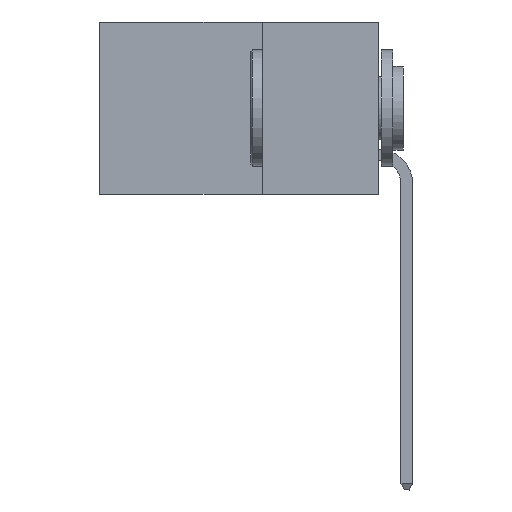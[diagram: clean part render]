
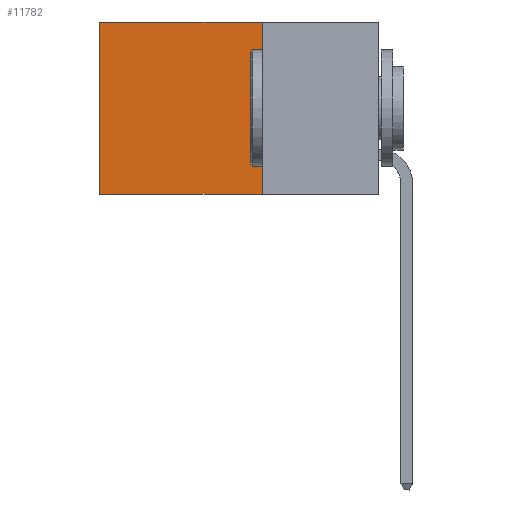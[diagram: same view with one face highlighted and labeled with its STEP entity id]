
A CAD part, left-side view. The second image highlights one B-rep face of the part: STEP entity #11782.
In plain terms, the highlighted planar face has unit normal (-1, 0, 0).
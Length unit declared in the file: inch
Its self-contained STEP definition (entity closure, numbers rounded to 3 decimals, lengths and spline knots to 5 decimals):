
#313 = LINE ( 'NONE', #8592, #5390 ) ;
#401 = PLANE ( 'NONE',  #14163 ) ;
#3255 = CARTESIAN_POINT ( 'NONE',  ( 0.2615, 0.6, 0. ) ) ;
#3264 = ORIENTED_EDGE ( 'NONE', *, *, #5200, .F. ) ;
#4010 = ORIENTED_EDGE ( 'NONE', *, *, #9057, .T. ) ;
#4093 = DIRECTION ( 'NONE',  ( 1., 0., 0. ) ) ;
#4376 = CARTESIAN_POINT ( 'NONE',  ( 0.2615, 0.25, -0.37 ) ) ;
#4456 = DIRECTION ( 'NONE',  ( 0., 0., -1. ) ) ;
#4638 = LINE ( 'NONE', #4376, #11140 ) ;
#5200 = EDGE_CURVE ( 'NONE', #15644, #7319, #11091, .T. ) ;
#5311 = CARTESIAN_POINT ( 'NONE',  ( 0.2615, 0.25, -0.37 ) ) ;
#5390 = VECTOR ( 'NONE', #16894, 39.37008 ) ;
#7319 = VERTEX_POINT ( 'NONE', #5311 ) ;
#7601 = VERTEX_POINT ( 'NONE', #16983 ) ;
#8563 = DIRECTION ( 'NONE',  ( 0., 1., 0. ) ) ;
#8592 = CARTESIAN_POINT ( 'NONE',  ( 0.2615, 0.6, -0.37 ) ) ;
#9057 = EDGE_CURVE ( 'NONE', #10696, #7601, #313, .T. ) ;
#10593 = EDGE_CURVE ( 'NONE', #7319, #7601, #4638, .T. ) ;
#10696 = VERTEX_POINT ( 'NONE', #3255 ) ;
#11091 = LINE ( 'NONE', #12986, #21634 ) ;
#11140 = VECTOR ( 'NONE', #8563, 39.37008 ) ;
#11782 = ADVANCED_FACE ( 'NONE', ( #16978 ), #401, .F. ) ;
#11790 = VECTOR ( 'NONE', #22629, 39.37008 ) ;
#12986 = CARTESIAN_POINT ( 'NONE',  ( 0.2615, 0.25, -0.37 ) ) ;
#14163 = AXIS2_PLACEMENT_3D ( 'NONE', #19044, #4093, #25041 ) ;
#15644 = VERTEX_POINT ( 'NONE', #25640 ) ;
#16894 = DIRECTION ( 'NONE',  ( 0., 0., -1. ) ) ;
#16978 = FACE_OUTER_BOUND ( 'NONE', #26842, .T. ) ;
#16983 = CARTESIAN_POINT ( 'NONE',  ( 0.2615, 0.6, -0.37 ) ) ;
#19044 = CARTESIAN_POINT ( 'NONE',  ( 0.2615, 0.25, -0.37 ) ) ;
#21634 = VECTOR ( 'NONE', #4456, 39.37008 ) ;
#21654 = EDGE_CURVE ( 'NONE', #15644, #10696, #22898, .T. ) ;
#22137 = ORIENTED_EDGE ( 'NONE', *, *, #10593, .F. ) ;
#22629 = DIRECTION ( 'NONE',  ( 0., 1., 0. ) ) ;
#22898 = LINE ( 'NONE', #26725, #11790 ) ;
#25041 = DIRECTION ( 'NONE',  ( 0., 0., -1. ) ) ;
#25633 = ORIENTED_EDGE ( 'NONE', *, *, #21654, .T. ) ;
#25640 = CARTESIAN_POINT ( 'NONE',  ( 0.2615, 0.25, 0. ) ) ;
#26725 = CARTESIAN_POINT ( 'NONE',  ( 0.2615, 0.25, 0. ) ) ;
#26842 = EDGE_LOOP ( 'NONE', ( #4010, #22137, #3264, #25633 ) ) ;
